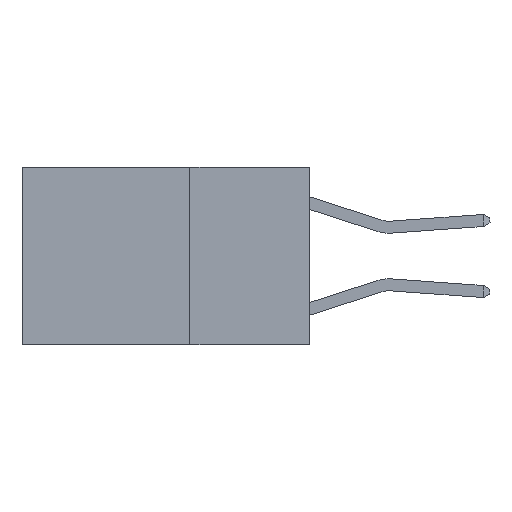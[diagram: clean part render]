
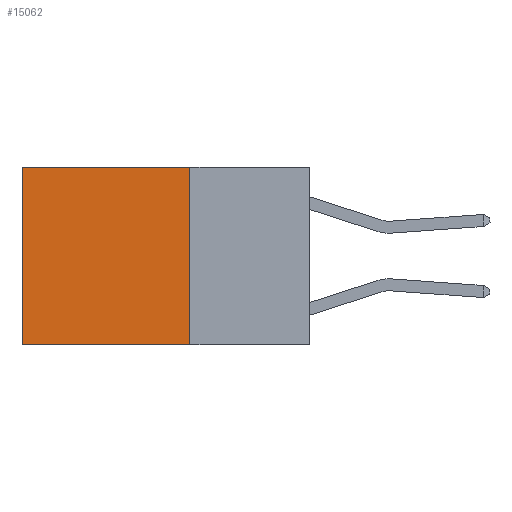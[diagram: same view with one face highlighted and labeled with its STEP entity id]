
A CAD part, left-side view. The second image highlights one B-rep face of the part: STEP entity #15062.
In plain terms, the highlighted planar face has unit normal (-1, 0, 0).
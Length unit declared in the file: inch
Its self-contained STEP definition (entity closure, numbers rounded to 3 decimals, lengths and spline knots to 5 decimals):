
#78 = LINE ( 'NONE', #14873, #13770 ) ;
#469 = DIRECTION ( 'NONE',  ( 0., 0., -1. ) ) ;
#513 = VERTEX_POINT ( 'NONE', #2591 ) ;
#1487 = LINE ( 'NONE', #16768, #13451 ) ;
#2591 = CARTESIAN_POINT ( 'NONE',  ( 0.2625, 0.25, -0.37 ) ) ;
#2893 = EDGE_CURVE ( 'NONE', #14448, #2925, #78, .T. ) ;
#2925 = VERTEX_POINT ( 'NONE', #8273 ) ;
#3150 = PLANE ( 'NONE',  #12256 ) ;
#3360 = DIRECTION ( 'NONE',  ( 0., 1., 0. ) ) ;
#3453 = VECTOR ( 'NONE', #13928, 39.37008 ) ;
#3571 = VERTEX_POINT ( 'NONE', #12007 ) ;
#4303 = LINE ( 'NONE', #4694, #3453 ) ;
#4694 = CARTESIAN_POINT ( 'NONE',  ( 0.2625, 0.25, 0. ) ) ;
#4716 = CARTESIAN_POINT ( 'NONE',  ( 0.2625, 0.25, -0.37 ) ) ;
#5398 = ORIENTED_EDGE ( 'NONE', *, *, #6573, .F. ) ;
#6573 = EDGE_CURVE ( 'NONE', #513, #3571, #10982, .T. ) ;
#7133 = EDGE_CURVE ( 'NONE', #14448, #513, #4303, .T. ) ;
#7447 = DIRECTION ( 'NONE',  ( 0., 1., 0. ) ) ;
#8273 = CARTESIAN_POINT ( 'NONE',  ( 0.2625, 0.6, 0. ) ) ;
#8565 = FACE_OUTER_BOUND ( 'NONE', #17012, .T. ) ;
#8650 = DIRECTION ( 'NONE',  ( 1., 0., 0. ) ) ;
#9041 = ORIENTED_EDGE ( 'NONE', *, *, #7133, .F. ) ;
#10158 = VECTOR ( 'NONE', #7447, 39.37008 ) ;
#10982 = LINE ( 'NONE', #4716, #10158 ) ;
#11519 = DIRECTION ( 'NONE',  ( 0., 0., -1. ) ) ;
#11872 = CARTESIAN_POINT ( 'NONE',  ( 0.2625, 0.25, 0. ) ) ;
#12007 = CARTESIAN_POINT ( 'NONE',  ( 0.2625, 0.6, -0.37 ) ) ;
#12256 = AXIS2_PLACEMENT_3D ( 'NONE', #16410, #8650, #469 ) ;
#13451 = VECTOR ( 'NONE', #11519, 39.37008 ) ;
#13770 = VECTOR ( 'NONE', #3360, 39.37008 ) ;
#13928 = DIRECTION ( 'NONE',  ( 0., 0., -1. ) ) ;
#14448 = VERTEX_POINT ( 'NONE', #11872 ) ;
#14692 = ORIENTED_EDGE ( 'NONE', *, *, #2893, .T. ) ;
#14873 = CARTESIAN_POINT ( 'NONE',  ( 0.2625, 0.25, 0. ) ) ;
#15062 = ADVANCED_FACE ( 'NONE', ( #8565 ), #3150, .F. ) ;
#16231 = ORIENTED_EDGE ( 'NONE', *, *, #17060, .T. ) ;
#16410 = CARTESIAN_POINT ( 'NONE',  ( 0.2625, 0.25, 0. ) ) ;
#16768 = CARTESIAN_POINT ( 'NONE',  ( 0.2625, 0.6, 0. ) ) ;
#17012 = EDGE_LOOP ( 'NONE', ( #16231, #5398, #9041, #14692 ) ) ;
#17060 = EDGE_CURVE ( 'NONE', #2925, #3571, #1487, .T. ) ;
